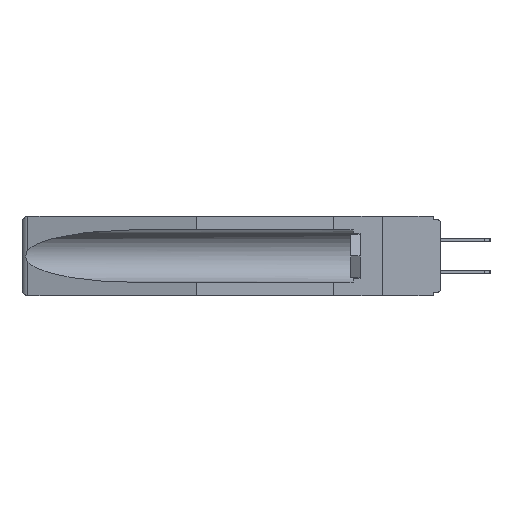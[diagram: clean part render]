
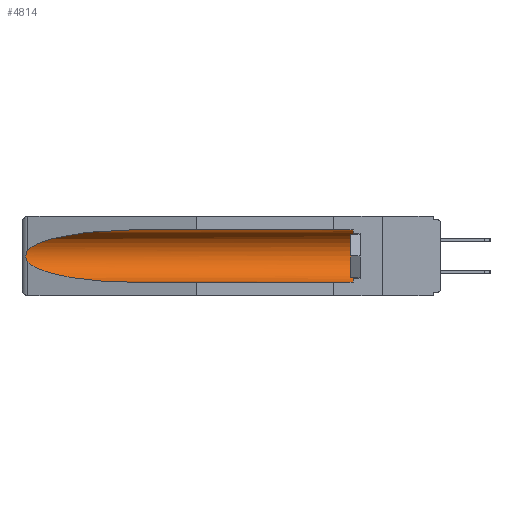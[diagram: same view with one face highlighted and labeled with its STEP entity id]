
A CAD part, left-side view. The second image highlights one B-rep face of the part: STEP entity #4814.
In plain terms, the highlighted cylindrical face has radius 2.857 mm (diameter 5.715 mm), a partial arc.
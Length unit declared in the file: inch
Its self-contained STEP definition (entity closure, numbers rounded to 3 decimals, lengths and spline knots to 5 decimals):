
#933 = CARTESIAN_POINT ( 'NONE',  ( 0.155, 0.126, -0.1715 ) ) ;
#1781 = CARTESIAN_POINT ( 'NONE',  ( 0.155, -0.30754, -0.284 ) ) ;
#1875 = CARTESIAN_POINT ( 'NONE',  ( 0.25451, 1.48313, -0.09465 ) ) ;
#2226 = CARTESIAN_POINT ( 'NONE',  ( 0.2675, 1.53308, -0.16763 ) ) ;
#2504 = CARTESIAN_POINT ( 'NONE',  ( 0.26537, 1.52718, -0.19328 ) ) ;
#2602 = DIRECTION ( 'NONE',  ( 0., 0., 1. ) ) ;
#3141 = B_SPLINE_CURVE_WITH_KNOTS ( 'NONE', 3,
 ( #7917, #25689, #8500, #11037, #2226, #17674, #4444, #9076, #18121, #2504 ),
 .UNSPECIFIED., .F., .F.,
 ( 4, 2, 2, 2, 4 ),
 ( 0., 0.00029, 0.00058, 0.00087, 0.00117 ),
 .UNSPECIFIED. ) ;
#3168 = EDGE_CURVE ( 'NONE', #4113, #10894, #27821, .T. ) ;
#3762 = EDGE_CURVE ( 'NONE', #22279, #23667, #20138, .T. ) ;
#4113 = VERTEX_POINT ( 'NONE', #7530 ) ;
#4444 = CARTESIAN_POINT ( 'NONE',  ( 0.2673, 1.53269, -0.17917 ) ) ;
#4772 = AXIS2_PLACEMENT_3D ( 'NONE', #13367, #9176, #2602 ) ;
#4814 = ADVANCED_FACE ( 'NONE', ( #26410 ), #14306, .F. ) ;
#5082 = CARTESIAN_POINT ( 'NONE',  ( 0.155, 1.07973, -0.284 ) ) ;
#7107 = CARTESIAN_POINT ( 'NONE',  ( 0.26537, 1.52718, -0.19328 ) ) ;
#7530 = CARTESIAN_POINT ( 'NONE',  ( 0.155, 0.126, -0.059 ) ) ;
#7917 = CARTESIAN_POINT ( 'NONE',  ( 0.26537, 1.52718, -0.14972 ) ) ;
#8237 = CARTESIAN_POINT ( 'NONE',  ( 0.21114, 1.30732, -0.059 ) ) ;
#8500 = CARTESIAN_POINT ( 'NONE',  ( 0.26654, 1.53092, -0.15636 ) ) ;
#8701 = EDGE_CURVE ( 'NONE', #10894, #20241, #22088, .T. ) ;
#9076 = CARTESIAN_POINT ( 'NONE',  ( 0.26655, 1.53094, -0.18657 ) ) ;
#9176 = DIRECTION ( 'NONE',  ( 0., 1., 0. ) ) ;
#9230 = CARTESIAN_POINT ( 'NONE',  ( 0.155, 1.07973, -0.284 ) ) ;
#9315 = ORIENTED_EDGE ( 'NONE', *, *, #15081, .T. ) ;
#9518 = VECTOR ( 'NONE', #27492, 39.37008 ) ;
#10796 = CIRCLE ( 'NONE', #24511, 0.1125 ) ;
#10894 = VERTEX_POINT ( 'NONE', #25704 ) ;
#11037 = CARTESIAN_POINT ( 'NONE',  ( 0.2673, 1.5327, -0.16383 ) ) ;
#13034 = VERTEX_POINT ( 'NONE', #19757 ) ;
#13367 = CARTESIAN_POINT ( 'NONE',  ( 0.155, -0.30754, -0.1715 ) ) ;
#13397 = ORIENTED_EDGE ( 'NONE', *, *, #24056, .T. ) ;
#13795 = CARTESIAN_POINT ( 'NONE',  ( 0.21114, 1.30732, -0.284 ) ) ;
#13819 = ORIENTED_EDGE ( 'NONE', *, *, #3762, .F. ) ;
#14306 = CYLINDRICAL_SURFACE ( 'NONE', #4772, 0.1125 ) ;
#14559 = EDGE_LOOP ( 'NONE', ( #17020, #9315, #19453, #13819, #13397, #19427 ) ) ;
#15081 = EDGE_CURVE ( 'NONE', #20241, #13034, #3141, .T. ) ;
#16509 = CARTESIAN_POINT ( 'NONE',  ( 0.155, -0.30754, -0.059 ) ) ;
#17020 = ORIENTED_EDGE ( 'NONE', *, *, #8701, .T. ) ;
#17338 = CARTESIAN_POINT ( 'NONE',  ( 0.26537, 1.52718, -0.14972 ) ) ;
#17674 = CARTESIAN_POINT ( 'NONE',  ( 0.2675, 1.53308, -0.17534 ) ) ;
#18121 = CARTESIAN_POINT ( 'NONE',  ( 0.26597, 1.5296, -0.19026 ) ) ;
#18387 = DIRECTION ( 'NONE',  ( 0., -1., 0. ) ) ;
#18690 = CARTESIAN_POINT ( 'NONE',  ( 0.155, 0.126, -0.284 ) ) ;
#19427 = ORIENTED_EDGE ( 'NONE', *, *, #3168, .T. ) ;
#19453 = ORIENTED_EDGE ( 'NONE', *, *, #19815, .T. ) ;
#19757 = CARTESIAN_POINT ( 'NONE',  ( 0.26537, 1.52718, -0.19328 ) ) ;
#19815 = EDGE_CURVE ( 'NONE', #13034, #23667, #26701, .T. ) ;
#20138 = LINE ( 'NONE', #1781, #27077 ) ;
#20241 = VERTEX_POINT ( 'NONE', #25221 ) ;
#22088 =( BOUNDED_CURVE ( )  B_SPLINE_CURVE ( 3, ( #28028, #8237, #1875, #17338 ),
 .UNSPECIFIED., .F., .F. ) 
 B_SPLINE_CURVE_WITH_KNOTS ( ( 4, 4 ),
 ( 4.71239, 6.08839 ),
 .UNSPECIFIED. ) 
 CURVE ( )  GEOMETRIC_REPRESENTATION_ITEM ( )  RATIONAL_B_SPLINE_CURVE ( ( 1., 0.848, 0.848, 1. ) ) 
 REPRESENTATION_ITEM ( '' )  );
#22279 = VERTEX_POINT ( 'NONE', #18690 ) ;
#22930 = DIRECTION ( 'NONE',  ( 0., 0., 1. ) ) ;
#23667 = VERTEX_POINT ( 'NONE', #9230 ) ;
#23989 = DIRECTION ( 'NONE',  ( 0., 1., 0. ) ) ;
#24056 = EDGE_CURVE ( 'NONE', #22279, #4113, #10796, .T. ) ;
#24511 = AXIS2_PLACEMENT_3D ( 'NONE', #933, #18387, #22930 ) ;
#25221 = CARTESIAN_POINT ( 'NONE',  ( 0.26537, 1.52718, -0.14972 ) ) ;
#25689 = CARTESIAN_POINT ( 'NONE',  ( 0.26597, 1.52961, -0.15275 ) ) ;
#25704 = CARTESIAN_POINT ( 'NONE',  ( 0.155, 1.07973, -0.059 ) ) ;
#26410 = FACE_OUTER_BOUND ( 'NONE', #14559, .T. ) ;
#26701 =( BOUNDED_CURVE ( )  B_SPLINE_CURVE ( 3, ( #7107, #26987, #13795, #5082 ),
 .UNSPECIFIED., .F., .F. ) 
 B_SPLINE_CURVE_WITH_KNOTS ( ( 4, 4 ),
 ( 0.1948, 1.5708 ),
 .UNSPECIFIED. ) 
 CURVE ( )  GEOMETRIC_REPRESENTATION_ITEM ( )  RATIONAL_B_SPLINE_CURVE ( ( 1., 0.848, 0.848, 1. ) ) 
 REPRESENTATION_ITEM ( '' )  );
#26987 = CARTESIAN_POINT ( 'NONE',  ( 0.25451, 1.48313, -0.24835 ) ) ;
#27077 = VECTOR ( 'NONE', #23989, 39.37008 ) ;
#27492 = DIRECTION ( 'NONE',  ( 0., 1., 0. ) ) ;
#27821 = LINE ( 'NONE', #16509, #9518 ) ;
#28028 = CARTESIAN_POINT ( 'NONE',  ( 0.155, 1.07973, -0.059 ) ) ;
